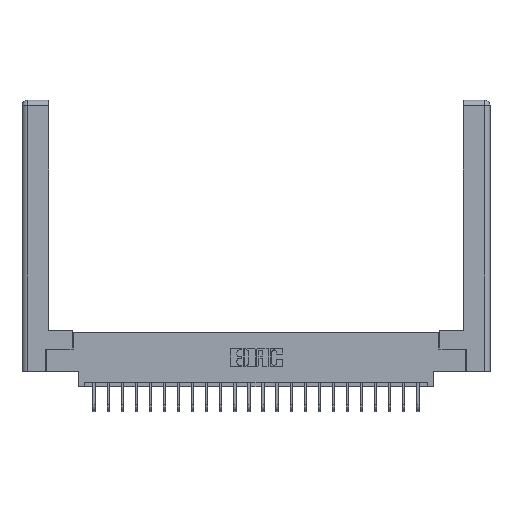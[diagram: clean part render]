
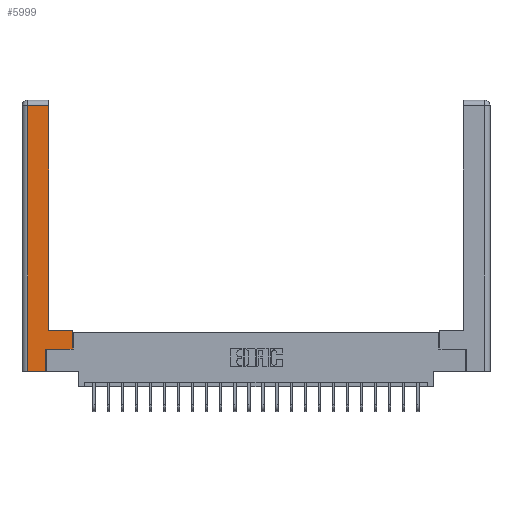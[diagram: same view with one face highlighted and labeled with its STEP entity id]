
A CAD part, top view. The second image highlights one B-rep face of the part: STEP entity #5999.
In plain terms, the highlighted planar face has unit normal (0, 0, 1).
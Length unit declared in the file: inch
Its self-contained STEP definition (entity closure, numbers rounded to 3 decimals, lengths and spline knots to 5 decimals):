
#94 = CARTESIAN_POINT ( 'NONE',  ( 0.265, 0., 0. ) ) ;
#156 = EDGE_CURVE ( 'NONE', #5559, #22540, #6708, .T. ) ;
#537 = ORIENTED_EDGE ( 'NONE', *, *, #5945, .T. ) ;
#661 = EDGE_CURVE ( 'NONE', #21639, #7762, #23970, .T. ) ;
#835 = ORIENTED_EDGE ( 'NONE', *, *, #156, .T. ) ;
#1499 = VECTOR ( 'NONE', #12361, 39.37008 ) ;
#1589 = DIRECTION ( 'NONE',  ( -1., 0., 0. ) ) ;
#1612 = PLANE ( 'NONE',  #2427 ) ;
#1705 = CARTESIAN_POINT ( 'NONE',  ( 0., 0., 0. ) ) ;
#2427 = AXIS2_PLACEMENT_3D ( 'NONE', #1705, #9604, #23013 ) ;
#2476 = VERTEX_POINT ( 'NONE', #5314 ) ;
#3370 = LINE ( 'NONE', #23471, #11677 ) ;
#3491 = CARTESIAN_POINT ( 'NONE',  ( 0.265, 0., 0. ) ) ;
#4051 = VECTOR ( 'NONE', #7597, 39.37008 ) ;
#4944 = DIRECTION ( 'NONE',  ( -1., 0., 0. ) ) ;
#5012 = ORIENTED_EDGE ( 'NONE', *, *, #24900, .T. ) ;
#5061 = LINE ( 'NONE', #24597, #11189 ) ;
#5314 = CARTESIAN_POINT ( 'NONE',  ( 0.0615, 2.94, 0. ) ) ;
#5335 = VERTEX_POINT ( 'NONE', #9513 ) ;
#5559 = VERTEX_POINT ( 'NONE', #94 ) ;
#5945 = EDGE_CURVE ( 'NONE', #22540, #21639, #20955, .T. ) ;
#5999 = ADVANCED_FACE ( 'NONE', ( #6201 ), #1612, .F. ) ;
#6072 = CARTESIAN_POINT ( 'NONE',  ( 0.295, 0.45, 0. ) ) ;
#6201 = FACE_OUTER_BOUND ( 'NONE', #24023, .T. ) ;
#6708 = LINE ( 'NONE', #17912, #1499 ) ;
#7597 = DIRECTION ( 'NONE',  ( 1., 0., 0. ) ) ;
#7762 = VERTEX_POINT ( 'NONE', #13886 ) ;
#8439 = CARTESIAN_POINT ( 'NONE',  ( 0.265, 0.245, 0. ) ) ;
#8726 = DIRECTION ( 'NONE',  ( 0., -1., 0. ) ) ;
#8817 = VECTOR ( 'NONE', #1589, 39.37008 ) ;
#9394 = CARTESIAN_POINT ( 'NONE',  ( 0.565, 0.245, 0. ) ) ;
#9513 = CARTESIAN_POINT ( 'NONE',  ( 0.295, 2.94, 0. ) ) ;
#9604 = DIRECTION ( 'NONE',  ( 0., 0., -1. ) ) ;
#10488 = EDGE_CURVE ( 'NONE', #7762, #25279, #5061, .T. ) ;
#11189 = VECTOR ( 'NONE', #4944, 39.37008 ) ;
#11677 = VECTOR ( 'NONE', #13446, 39.37008 ) ;
#11862 = CARTESIAN_POINT ( 'NONE',  ( 0.0615, 0., 0. ) ) ;
#12361 = DIRECTION ( 'NONE',  ( 0., 1., 0. ) ) ;
#12458 = ORIENTED_EDGE ( 'NONE', *, *, #25443, .T. ) ;
#13434 = EDGE_CURVE ( 'NONE', #5335, #2476, #15850, .T. ) ;
#13446 = DIRECTION ( 'NONE',  ( 0., 1., 0. ) ) ;
#13886 = CARTESIAN_POINT ( 'NONE',  ( 0.565, 0.45, 0. ) ) ;
#14403 = CARTESIAN_POINT ( 'NONE',  ( 0.565, 0.45, 0. ) ) ;
#14421 = VECTOR ( 'NONE', #16028, 39.37008 ) ;
#15850 = LINE ( 'NONE', #17020, #8817 ) ;
#15925 = VECTOR ( 'NONE', #18362, 39.37008 ) ;
#15971 = LINE ( 'NONE', #3491, #14421 ) ;
#16028 = DIRECTION ( 'NONE',  ( 1., 0., 0. ) ) ;
#16064 = ORIENTED_EDGE ( 'NONE', *, *, #661, .T. ) ;
#17020 = CARTESIAN_POINT ( 'NONE',  ( 0.0615, 2.94, 0. ) ) ;
#17912 = CARTESIAN_POINT ( 'NONE',  ( 0.265, 0.245, 0. ) ) ;
#18265 = EDGE_CURVE ( 'NONE', #25279, #5335, #3370, .T. ) ;
#18362 = DIRECTION ( 'NONE',  ( 0., 1., 0. ) ) ;
#18379 = VECTOR ( 'NONE', #8726, 39.37008 ) ;
#19018 = ORIENTED_EDGE ( 'NONE', *, *, #13434, .T. ) ;
#19150 = VERTEX_POINT ( 'NONE', #11862 ) ;
#20350 = ORIENTED_EDGE ( 'NONE', *, *, #18265, .T. ) ;
#20955 = LINE ( 'NONE', #9394, #4051 ) ;
#21639 = VERTEX_POINT ( 'NONE', #23395 ) ;
#22030 = ORIENTED_EDGE ( 'NONE', *, *, #10488, .T. ) ;
#22540 = VERTEX_POINT ( 'NONE', #8439 ) ;
#22861 = CARTESIAN_POINT ( 'NONE',  ( 0.0615, 0., 0. ) ) ;
#23013 = DIRECTION ( 'NONE',  ( -1., 0., 0. ) ) ;
#23395 = CARTESIAN_POINT ( 'NONE',  ( 0.565, 0.245, 0. ) ) ;
#23471 = CARTESIAN_POINT ( 'NONE',  ( 0.295, 3., 0. ) ) ;
#23970 = LINE ( 'NONE', #14403, #15925 ) ;
#24023 = EDGE_LOOP ( 'NONE', ( #20350, #19018, #12458, #5012, #835, #537, #16064, #22030 ) ) ;
#24300 = LINE ( 'NONE', #22861, #18379 ) ;
#24597 = CARTESIAN_POINT ( 'NONE',  ( 0.295, 0.45, 0. ) ) ;
#24900 = EDGE_CURVE ( 'NONE', #19150, #5559, #15971, .T. ) ;
#25279 = VERTEX_POINT ( 'NONE', #6072 ) ;
#25443 = EDGE_CURVE ( 'NONE', #2476, #19150, #24300, .T. ) ;
